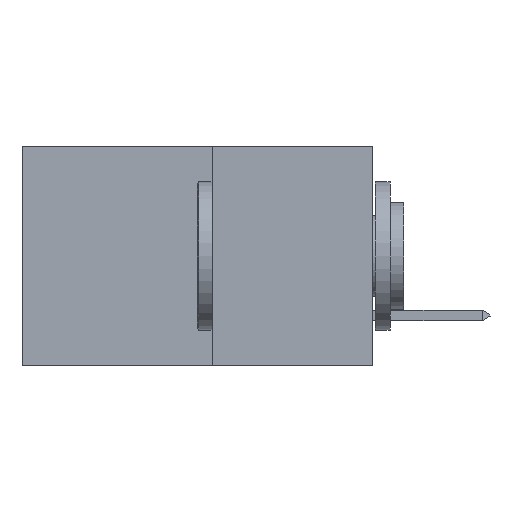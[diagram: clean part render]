
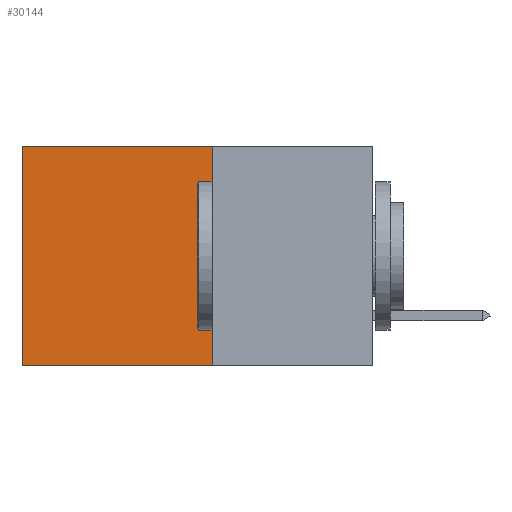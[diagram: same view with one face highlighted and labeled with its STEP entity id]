
A CAD part, left-side view. The second image highlights one B-rep face of the part: STEP entity #30144.
In plain terms, the highlighted planar face has unit normal (-1, 0, 0).
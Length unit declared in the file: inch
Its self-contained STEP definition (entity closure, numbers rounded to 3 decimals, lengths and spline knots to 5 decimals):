
#1076 = DIRECTION ( 'NONE',  ( 0., 1., 0. ) ) ;
#2114 = DIRECTION ( 'NONE',  ( 1., 0., 0. ) ) ;
#2647 = EDGE_CURVE ( 'NONE', #11370, #10389, #23841, .T. ) ;
#6740 = LINE ( 'NONE', #31628, #26226 ) ;
#8735 = VECTOR ( 'NONE', #15653, 39.37008 ) ;
#9553 = CARTESIAN_POINT ( 'NONE',  ( 0.277, 0.27, -0.37 ) ) ;
#9580 = VECTOR ( 'NONE', #13022, 39.37008 ) ;
#10389 = VERTEX_POINT ( 'NONE', #9553 ) ;
#11370 = VERTEX_POINT ( 'NONE', #20533 ) ;
#11511 = EDGE_CURVE ( 'NONE', #10389, #26325, #21043, .T. ) ;
#11838 = FACE_OUTER_BOUND ( 'NONE', #18438, .T. ) ;
#11915 = EDGE_CURVE ( 'NONE', #22479, #26325, #16688, .T. ) ;
#12496 = ORIENTED_EDGE ( 'NONE', *, *, #2647, .F. ) ;
#13022 = DIRECTION ( 'NONE',  ( 0., 0., -1. ) ) ;
#13920 = CARTESIAN_POINT ( 'NONE',  ( 0.277, 0.27, -0.37 ) ) ;
#15653 = DIRECTION ( 'NONE',  ( 0., 0., -1. ) ) ;
#16688 = LINE ( 'NONE', #21539, #9580 ) ;
#18438 = EDGE_LOOP ( 'NONE', ( #28424, #23591, #12496, #24806 ) ) ;
#18458 = DIRECTION ( 'NONE',  ( 0., 1., 0. ) ) ;
#19959 = DIRECTION ( 'NONE',  ( 0., 0., -1. ) ) ;
#20533 = CARTESIAN_POINT ( 'NONE',  ( 0.277, 0.27, 0. ) ) ;
#21043 = LINE ( 'NONE', #31235, #27034 ) ;
#21539 = CARTESIAN_POINT ( 'NONE',  ( 0.277, 0.59, -0.37 ) ) ;
#22479 = VERTEX_POINT ( 'NONE', #25795 ) ;
#23591 = ORIENTED_EDGE ( 'NONE', *, *, #11511, .F. ) ;
#23841 = LINE ( 'NONE', #13920, #8735 ) ;
#24806 = ORIENTED_EDGE ( 'NONE', *, *, #28580, .T. ) ;
#25795 = CARTESIAN_POINT ( 'NONE',  ( 0.277, 0.59, 0. ) ) ;
#25811 = CARTESIAN_POINT ( 'NONE',  ( 0.277, 0.59, -0.37 ) ) ;
#26226 = VECTOR ( 'NONE', #1076, 39.37008 ) ;
#26325 = VERTEX_POINT ( 'NONE', #25811 ) ;
#27034 = VECTOR ( 'NONE', #18458, 39.37008 ) ;
#28424 = ORIENTED_EDGE ( 'NONE', *, *, #11915, .T. ) ;
#28580 = EDGE_CURVE ( 'NONE', #11370, #22479, #6740, .T. ) ;
#30089 = PLANE ( 'NONE',  #30733 ) ;
#30144 = ADVANCED_FACE ( 'NONE', ( #11838 ), #30089, .F. ) ;
#30733 = AXIS2_PLACEMENT_3D ( 'NONE', #32643, #2114, #19959 ) ;
#31235 = CARTESIAN_POINT ( 'NONE',  ( 0.277, 0.27, -0.37 ) ) ;
#31628 = CARTESIAN_POINT ( 'NONE',  ( 0.277, 0.27, 0. ) ) ;
#32643 = CARTESIAN_POINT ( 'NONE',  ( 0.277, 0.27, -0.37 ) ) ;
